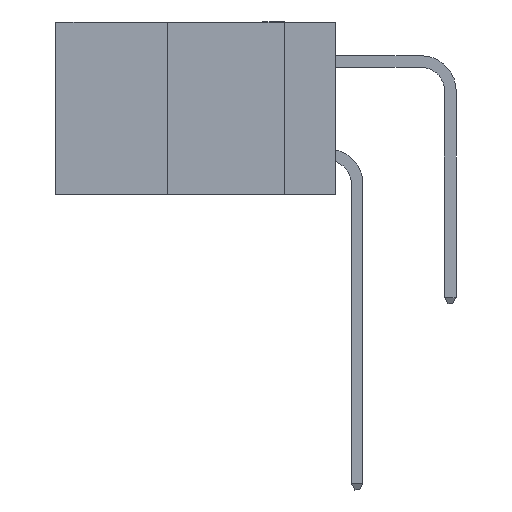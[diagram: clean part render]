
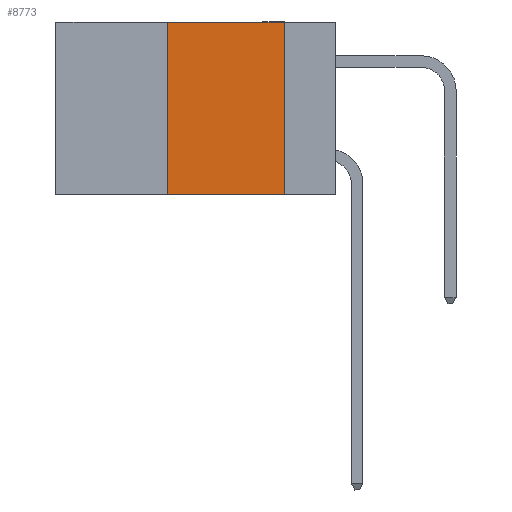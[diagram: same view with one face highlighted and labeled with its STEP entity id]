
A CAD part, left-side view. The second image highlights one B-rep face of the part: STEP entity #8773.
In plain terms, the highlighted planar face has unit normal (-1, 0, 0).
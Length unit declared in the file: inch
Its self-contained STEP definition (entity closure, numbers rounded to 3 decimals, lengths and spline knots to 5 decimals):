
#764 = EDGE_CURVE ( 'NONE', #16526, #8975, #7438, .T. ) ;
#820 = ORIENTED_EDGE ( 'NONE', *, *, #4607, .T. ) ;
#1273 = CARTESIAN_POINT ( 'NONE',  ( 0., 0.6, -0.37 ) ) ;
#2263 = VECTOR ( 'NONE', #7110, 39.37008 ) ;
#2288 = PLANE ( 'NONE',  #17331 ) ;
#3085 = VECTOR ( 'NONE', #6883, 39.37008 ) ;
#3597 = VECTOR ( 'NONE', #4889, 39.37008 ) ;
#4607 = EDGE_CURVE ( 'NONE', #16526, #12155, #15850, .T. ) ;
#4889 = DIRECTION ( 'NONE',  ( 0., 0., 1. ) ) ;
#5812 = ORIENTED_EDGE ( 'NONE', *, *, #17159, .F. ) ;
#6036 = VERTEX_POINT ( 'NONE', #15350 ) ;
#6459 = CARTESIAN_POINT ( 'NONE',  ( 0., 0.11, -0.37 ) ) ;
#6708 = ORIENTED_EDGE ( 'NONE', *, *, #764, .F. ) ;
#6774 = LINE ( 'NONE', #16472, #3085 ) ;
#6883 = DIRECTION ( 'NONE',  ( 0., -1., 0. ) ) ;
#7110 = DIRECTION ( 'NONE',  ( 0., -1., 0. ) ) ;
#7114 = EDGE_LOOP ( 'NONE', ( #13617, #5812, #6708, #820 ) ) ;
#7438 = LINE ( 'NONE', #10388, #3597 ) ;
#7653 = LINE ( 'NONE', #17487, #10858 ) ;
#8372 = CARTESIAN_POINT ( 'NONE',  ( 0., 0.36, -0.37 ) ) ;
#8773 = ADVANCED_FACE ( 'NONE', ( #17028 ), #2288, .F. ) ;
#8975 = VERTEX_POINT ( 'NONE', #13929 ) ;
#9041 = DIRECTION ( 'NONE',  ( 0., 0., -1. ) ) ;
#10388 = CARTESIAN_POINT ( 'NONE',  ( 0., 0.36, 0. ) ) ;
#10520 = DIRECTION ( 'NONE',  ( 0., 0., -1. ) ) ;
#10858 = VECTOR ( 'NONE', #9041, 39.37008 ) ;
#12155 = VERTEX_POINT ( 'NONE', #6459 ) ;
#13617 = ORIENTED_EDGE ( 'NONE', *, *, #16848, .F. ) ;
#13929 = CARTESIAN_POINT ( 'NONE',  ( 0., 0.36, 0. ) ) ;
#14514 = CARTESIAN_POINT ( 'NONE',  ( 0., 0.6, 0. ) ) ;
#15350 = CARTESIAN_POINT ( 'NONE',  ( 0., 0.11, 0. ) ) ;
#15850 = LINE ( 'NONE', #1273, #2263 ) ;
#15904 = DIRECTION ( 'NONE',  ( 1., 0., 0. ) ) ;
#16472 = CARTESIAN_POINT ( 'NONE',  ( 0., 0.6, 0. ) ) ;
#16526 = VERTEX_POINT ( 'NONE', #8372 ) ;
#16848 = EDGE_CURVE ( 'NONE', #6036, #12155, #7653, .T. ) ;
#17028 = FACE_OUTER_BOUND ( 'NONE', #7114, .T. ) ;
#17159 = EDGE_CURVE ( 'NONE', #8975, #6036, #6774, .T. ) ;
#17331 = AXIS2_PLACEMENT_3D ( 'NONE', #14514, #15904, #10520 ) ;
#17487 = CARTESIAN_POINT ( 'NONE',  ( 0., 0.11, 0. ) ) ;
